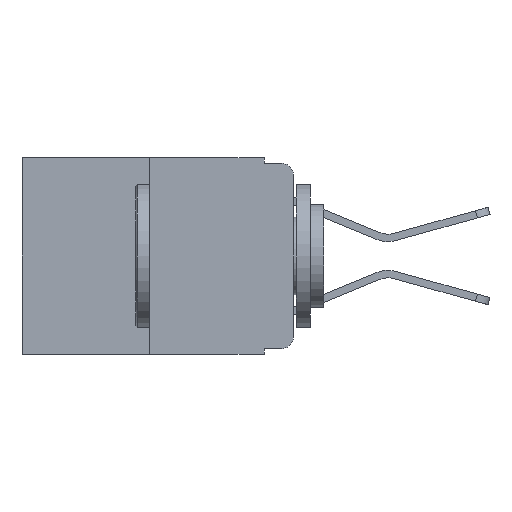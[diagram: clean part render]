
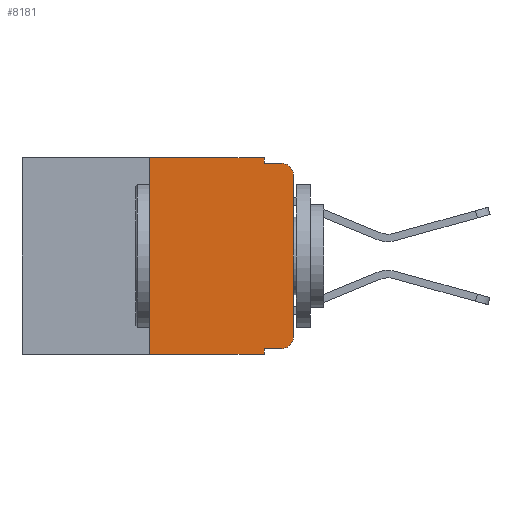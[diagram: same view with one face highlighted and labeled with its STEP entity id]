
A CAD part, left-side view. The second image highlights one B-rep face of the part: STEP entity #8181.
In plain terms, the highlighted planar face has unit normal (-1, 0, 0).
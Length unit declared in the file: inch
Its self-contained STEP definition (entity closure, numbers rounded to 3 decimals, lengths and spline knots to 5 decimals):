
#130 = CARTESIAN_POINT ( 'NONE',  ( 0., 0., -0.313 ) ) ;
#380 = DIRECTION ( 'NONE',  ( 0., 0., -1. ) ) ;
#463 = EDGE_CURVE ( 'NONE', #2370, #1049, #6689, .T. ) ;
#1049 = VERTEX_POINT ( 'NONE', #130 ) ;
#1162 = EDGE_CURVE ( 'NONE', #11604, #2370, #9608, .T. ) ;
#1274 = ORIENTED_EDGE ( 'NONE', *, *, #2648, .F. ) ;
#1719 = CARTESIAN_POINT ( 'NONE',  ( 0., 0.051, -0.343 ) ) ;
#1743 = EDGE_CURVE ( 'NONE', #3244, #7181, #7101, .T. ) ;
#1841 = LINE ( 'NONE', #4398, #9164 ) ;
#1933 = DIRECTION ( 'NONE',  ( -1., 0., 0. ) ) ;
#2080 = DIRECTION ( 'NONE',  ( 0., 0., 1. ) ) ;
#2112 = VECTOR ( 'NONE', #9960, 39.37008 ) ;
#2150 = CARTESIAN_POINT ( 'NONE',  ( 0., 0.051, -0.333 ) ) ;
#2305 = CARTESIAN_POINT ( 'NONE',  ( 0., 0.473, 0. ) ) ;
#2370 = VERTEX_POINT ( 'NONE', #10069 ) ;
#2648 = EDGE_CURVE ( 'NONE', #11604, #2803, #5812, .T. ) ;
#2663 = VERTEX_POINT ( 'NONE', #7227 ) ;
#2796 = DIRECTION ( 'NONE',  ( 1., 0., 0. ) ) ;
#2803 = VERTEX_POINT ( 'NONE', #1719 ) ;
#3123 = ORIENTED_EDGE ( 'NONE', *, *, #3309, .F. ) ;
#3194 = VERTEX_POINT ( 'NONE', #9898 ) ;
#3244 = VERTEX_POINT ( 'NONE', #8671 ) ;
#3309 = EDGE_CURVE ( 'NONE', #6192, #3244, #10797, .T. ) ;
#3420 = CARTESIAN_POINT ( 'NONE',  ( 0., 0.051, 0. ) ) ;
#3892 = ORIENTED_EDGE ( 'NONE', *, *, #8336, .T. ) ;
#4125 = AXIS2_PLACEMENT_3D ( 'NONE', #6408, #6177, #380 ) ;
#4398 = CARTESIAN_POINT ( 'NONE',  ( 0., 0.473, -0.343 ) ) ;
#4927 = ORIENTED_EDGE ( 'NONE', *, *, #10161, .T. ) ;
#5066 = ORIENTED_EDGE ( 'NONE', *, *, #5846, .F. ) ;
#5331 = CARTESIAN_POINT ( 'NONE',  ( 0., 0.051, -0.01 ) ) ;
#5645 = CARTESIAN_POINT ( 'NONE',  ( 0., 0.473, 0. ) ) ;
#5812 = LINE ( 'NONE', #6983, #8270 ) ;
#5846 = EDGE_CURVE ( 'NONE', #7181, #2663, #12025, .T. ) ;
#6177 = DIRECTION ( 'NONE',  ( -1., 0., 0. ) ) ;
#6192 = VERTEX_POINT ( 'NONE', #8649 ) ;
#6408 = CARTESIAN_POINT ( 'NONE',  ( 0., 0.02, -0.313 ) ) ;
#6438 = EDGE_CURVE ( 'NONE', #2663, #7934, #12142, .T. ) ;
#6689 = CIRCLE ( 'NONE', #4125, 0.02 ) ;
#6776 = AXIS2_PLACEMENT_3D ( 'NONE', #5645, #2796, #9362 ) ;
#6983 = CARTESIAN_POINT ( 'NONE',  ( 0., 0.051, 0. ) ) ;
#7101 = LINE ( 'NONE', #2305, #11642 ) ;
#7112 = VECTOR ( 'NONE', #7836, 39.37008 ) ;
#7169 = DIRECTION ( 'NONE',  ( 0., 0., -1. ) ) ;
#7181 = VERTEX_POINT ( 'NONE', #10047 ) ;
#7227 = CARTESIAN_POINT ( 'NONE',  ( 0., 0.051, -0.01 ) ) ;
#7325 = CARTESIAN_POINT ( 'NONE',  ( 0., 0.25, 0. ) ) ;
#7432 = PLANE ( 'NONE',  #6776 ) ;
#7657 = CARTESIAN_POINT ( 'NONE',  ( 0., 0.02, -0.03 ) ) ;
#7836 = DIRECTION ( 'NONE',  ( 0., -1., 0. ) ) ;
#7934 = VERTEX_POINT ( 'NONE', #9894 ) ;
#8181 = ADVANCED_FACE ( 'NONE', ( #11804 ), #7432, .F. ) ;
#8270 = VECTOR ( 'NONE', #7169, 39.37008 ) ;
#8314 = CIRCLE ( 'NONE', #11667, 0.02 ) ;
#8336 = EDGE_CURVE ( 'NONE', #3194, #7934, #8314, .T. ) ;
#8408 = VECTOR ( 'NONE', #8725, 39.37008 ) ;
#8624 = DIRECTION ( 'NONE',  ( 0., 0., -1. ) ) ;
#8649 = CARTESIAN_POINT ( 'NONE',  ( 0., 0.25, -0.343 ) ) ;
#8671 = CARTESIAN_POINT ( 'NONE',  ( 0., 0.25, 0. ) ) ;
#8725 = DIRECTION ( 'NONE',  ( 0., 0., 1. ) ) ;
#8752 = CARTESIAN_POINT ( 'NONE',  ( 0., 0., 0. ) ) ;
#8786 = EDGE_LOOP ( 'NONE', ( #4927, #3892, #9419, #5066, #12304, #3123, #11091, #1274, #9267, #11892 ) ) ;
#8897 = CARTESIAN_POINT ( 'NONE',  ( 0., 0.051, -0.333 ) ) ;
#9043 = DIRECTION ( 'NONE',  ( 0., -1., 0. ) ) ;
#9108 = EDGE_CURVE ( 'NONE', #6192, #2803, #1841, .T. ) ;
#9164 = VECTOR ( 'NONE', #10806, 39.37008 ) ;
#9233 = DIRECTION ( 'NONE',  ( 0., -1., 0. ) ) ;
#9267 = ORIENTED_EDGE ( 'NONE', *, *, #1162, .T. ) ;
#9362 = DIRECTION ( 'NONE',  ( 0., 0., -1. ) ) ;
#9419 = ORIENTED_EDGE ( 'NONE', *, *, #6438, .F. ) ;
#9458 = LINE ( 'NONE', #8752, #11500 ) ;
#9608 = LINE ( 'NONE', #2150, #7112 ) ;
#9797 = VECTOR ( 'NONE', #9043, 39.37008 ) ;
#9894 = CARTESIAN_POINT ( 'NONE',  ( 0., 0.02, -0.01 ) ) ;
#9898 = CARTESIAN_POINT ( 'NONE',  ( 0., 0., -0.03 ) ) ;
#9960 = DIRECTION ( 'NONE',  ( 0., 0., -1. ) ) ;
#10047 = CARTESIAN_POINT ( 'NONE',  ( 0., 0.051, 0. ) ) ;
#10069 = CARTESIAN_POINT ( 'NONE',  ( 0., 0.02, -0.333 ) ) ;
#10161 = EDGE_CURVE ( 'NONE', #1049, #3194, #9458, .T. ) ;
#10797 = LINE ( 'NONE', #7325, #8408 ) ;
#10806 = DIRECTION ( 'NONE',  ( 0., -1., 0. ) ) ;
#11091 = ORIENTED_EDGE ( 'NONE', *, *, #9108, .T. ) ;
#11500 = VECTOR ( 'NONE', #2080, 39.37008 ) ;
#11604 = VERTEX_POINT ( 'NONE', #8897 ) ;
#11642 = VECTOR ( 'NONE', #9233, 39.37008 ) ;
#11667 = AXIS2_PLACEMENT_3D ( 'NONE', #7657, #1933, #8624 ) ;
#11804 = FACE_OUTER_BOUND ( 'NONE', #8786, .T. ) ;
#11892 = ORIENTED_EDGE ( 'NONE', *, *, #463, .T. ) ;
#12025 = LINE ( 'NONE', #3420, #2112 ) ;
#12142 = LINE ( 'NONE', #5331, #9797 ) ;
#12304 = ORIENTED_EDGE ( 'NONE', *, *, #1743, .F. ) ;
